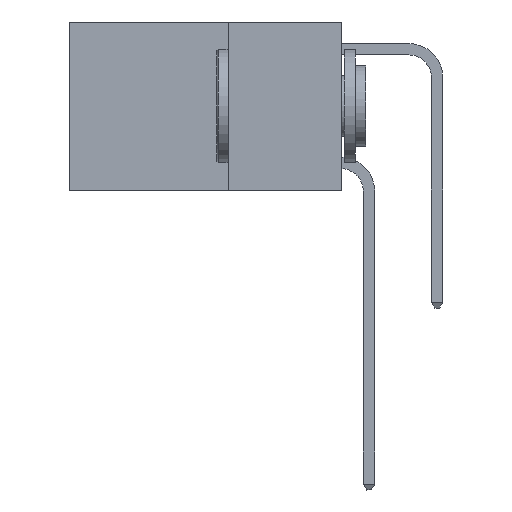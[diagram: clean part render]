
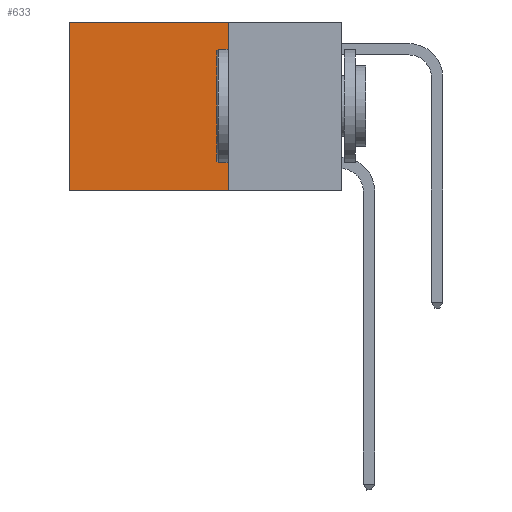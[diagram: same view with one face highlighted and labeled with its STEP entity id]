
A CAD part, left-side view. The second image highlights one B-rep face of the part: STEP entity #633.
In plain terms, the highlighted planar face has unit normal (-1, 0, 0).
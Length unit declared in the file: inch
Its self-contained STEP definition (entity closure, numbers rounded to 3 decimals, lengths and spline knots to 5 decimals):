
#547 = CARTESIAN_POINT ( 'NONE',  ( 0.2625, 0.25, 0. ) ) ;
#633 = ADVANCED_FACE ( 'NONE', ( #16226 ), #6392, .F. ) ;
#724 = ORIENTED_EDGE ( 'NONE', *, *, #4897, .T. ) ;
#1180 = AXIS2_PLACEMENT_3D ( 'NONE', #9387, #16041, #3655 ) ;
#2221 = LINE ( 'NONE', #14338, #15097 ) ;
#2609 = CARTESIAN_POINT ( 'NONE',  ( 0.2625, 0.25, -0.37 ) ) ;
#3655 = DIRECTION ( 'NONE',  ( 0., 0., -1. ) ) ;
#4897 = EDGE_CURVE ( 'NONE', #10863, #13671, #9945, .T. ) ;
#5044 = ORIENTED_EDGE ( 'NONE', *, *, #13690, .T. ) ;
#5408 = LINE ( 'NONE', #16324, #16120 ) ;
#5721 = CARTESIAN_POINT ( 'NONE',  ( 0.2625, 0.25, -0.37 ) ) ;
#6392 = PLANE ( 'NONE',  #1180 ) ;
#6597 = EDGE_LOOP ( 'NONE', ( #724, #12888, #14728, #5044 ) ) ;
#8182 = DIRECTION ( 'NONE',  ( 0., 0., -1. ) ) ;
#8679 = VERTEX_POINT ( 'NONE', #2609 ) ;
#9387 = CARTESIAN_POINT ( 'NONE',  ( 0.2625, 0.25, 0. ) ) ;
#9759 = VECTOR ( 'NONE', #11237, 39.37008 ) ;
#9945 = LINE ( 'NONE', #13745, #10838 ) ;
#10703 = EDGE_CURVE ( 'NONE', #8679, #13671, #14218, .T. ) ;
#10838 = VECTOR ( 'NONE', #8182, 39.37008 ) ;
#10863 = VERTEX_POINT ( 'NONE', #16189 ) ;
#10945 = DIRECTION ( 'NONE',  ( 0., 1., 0. ) ) ;
#11237 = DIRECTION ( 'NONE',  ( 0., 1., 0. ) ) ;
#12888 = ORIENTED_EDGE ( 'NONE', *, *, #10703, .F. ) ;
#12996 = DIRECTION ( 'NONE',  ( 0., 0., -1. ) ) ;
#13671 = VERTEX_POINT ( 'NONE', #17688 ) ;
#13690 = EDGE_CURVE ( 'NONE', #14361, #10863, #5408, .T. ) ;
#13745 = CARTESIAN_POINT ( 'NONE',  ( 0.2625, 0.6, 0. ) ) ;
#14218 = LINE ( 'NONE', #5721, #9759 ) ;
#14338 = CARTESIAN_POINT ( 'NONE',  ( 0.2625, 0.25, 0. ) ) ;
#14361 = VERTEX_POINT ( 'NONE', #547 ) ;
#14728 = ORIENTED_EDGE ( 'NONE', *, *, #17586, .F. ) ;
#15097 = VECTOR ( 'NONE', #12996, 39.37008 ) ;
#16041 = DIRECTION ( 'NONE',  ( 1., 0., 0. ) ) ;
#16120 = VECTOR ( 'NONE', #10945, 39.37008 ) ;
#16189 = CARTESIAN_POINT ( 'NONE',  ( 0.2625, 0.6, 0. ) ) ;
#16226 = FACE_OUTER_BOUND ( 'NONE', #6597, .T. ) ;
#16324 = CARTESIAN_POINT ( 'NONE',  ( 0.2625, 0.25, 0. ) ) ;
#17586 = EDGE_CURVE ( 'NONE', #14361, #8679, #2221, .T. ) ;
#17688 = CARTESIAN_POINT ( 'NONE',  ( 0.2625, 0.6, -0.37 ) ) ;
